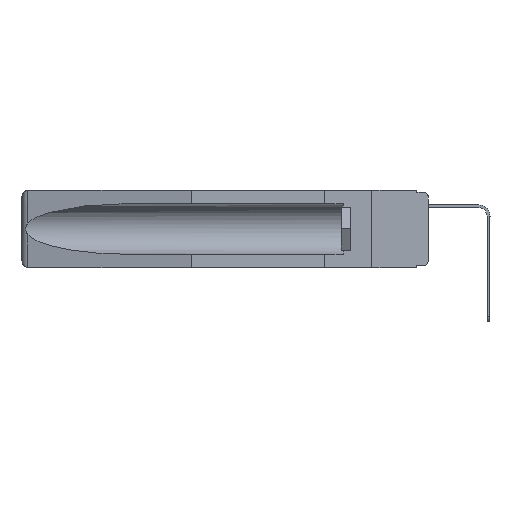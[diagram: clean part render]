
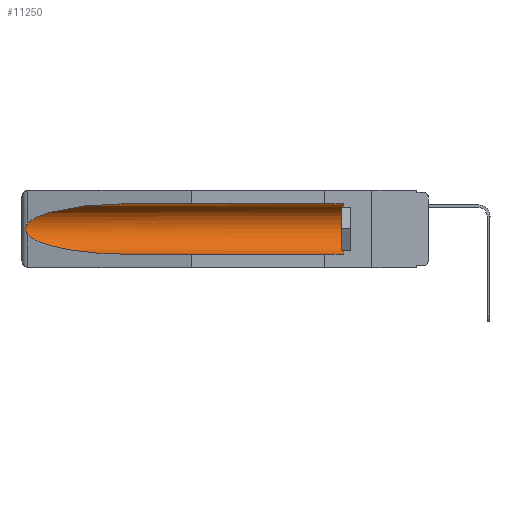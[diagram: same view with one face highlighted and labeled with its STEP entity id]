
A CAD part, left-side view. The second image highlights one B-rep face of the part: STEP entity #11250.
In plain terms, the highlighted cylindrical face has radius 2.857 mm (diameter 5.715 mm), a partial arc.
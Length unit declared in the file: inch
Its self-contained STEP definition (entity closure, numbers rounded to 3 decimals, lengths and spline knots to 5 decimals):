
#95 = EDGE_CURVE ( 'NONE', #7222, #11001, #99, .T. ) ;
#99 =( BOUNDED_CURVE ( )  B_SPLINE_CURVE ( 3, ( #16822, #16918, #8422, #4584 ),
 .UNSPECIFIED., .F., .F. ) 
 B_SPLINE_CURVE_WITH_KNOTS ( ( 4, 4 ),
 ( 4.71239, 6.08839 ),
 .UNSPECIFIED. ) 
 CURVE ( )  GEOMETRIC_REPRESENTATION_ITEM ( )  RATIONAL_B_SPLINE_CURVE ( ( 1., 0.848, 0.848, 1. ) ) 
 REPRESENTATION_ITEM ( '' )  );
#2267 = CARTESIAN_POINT ( 'NONE',  ( 0.155, 0.126, -0.1715 ) ) ;
#2500 = VECTOR ( 'NONE', #25527, 39.37008 ) ;
#2703 = DIRECTION ( 'NONE',  ( 0., 1., 0. ) ) ;
#2849 = CARTESIAN_POINT ( 'NONE',  ( 0.2673, 1.5327, -0.16383 ) ) ;
#3856 = ORIENTED_EDGE ( 'NONE', *, *, #95, .T. ) ;
#4128 = LINE ( 'NONE', #4716, #2500 ) ;
#4533 = EDGE_CURVE ( 'NONE', #25367, #26791, #5265, .T. ) ;
#4584 = CARTESIAN_POINT ( 'NONE',  ( 0.26537, 1.52718, -0.14972 ) ) ;
#4716 = CARTESIAN_POINT ( 'NONE',  ( 0.155, -0.30754, -0.059 ) ) ;
#4916 = CARTESIAN_POINT ( 'NONE',  ( 0.2675, 1.53308, -0.17534 ) ) ;
#5265 = LINE ( 'NONE', #25731, #25016 ) ;
#5566 = VERTEX_POINT ( 'NONE', #25139 ) ;
#6490 = EDGE_CURVE ( 'NONE', #25367, #23453, #13890, .T. ) ;
#7222 = VERTEX_POINT ( 'NONE', #23536 ) ;
#7542 = ORIENTED_EDGE ( 'NONE', *, *, #21500, .T. ) ;
#7669 = CARTESIAN_POINT ( 'NONE',  ( 0.25451, 1.48313, -0.24835 ) ) ;
#7683 = EDGE_CURVE ( 'NONE', #23453, #7222, #4128, .T. ) ;
#7862 = B_SPLINE_CURVE_WITH_KNOTS ( 'NONE', 3,
 ( #25556, #15195, #11122, #2849, #17074, #4916, #11203, #19445, #17253, #19168 ),
 .UNSPECIFIED., .F., .F.,
 ( 4, 2, 2, 2, 4 ),
 ( 0., 0.00029, 0.00058, 0.00087, 0.00117 ),
 .UNSPECIFIED. ) ;
#8422 = CARTESIAN_POINT ( 'NONE',  ( 0.25451, 1.48313, -0.09465 ) ) ;
#8702 = CARTESIAN_POINT ( 'NONE',  ( 0.155, 1.07973, -0.284 ) ) ;
#10171 = AXIS2_PLACEMENT_3D ( 'NONE', #21479, #2703, #23297 ) ;
#10248 = ORIENTED_EDGE ( 'NONE', *, *, #4533, .F. ) ;
#11001 = VERTEX_POINT ( 'NONE', #16662 ) ;
#11111 = CARTESIAN_POINT ( 'NONE',  ( 0.155, 0.126, -0.059 ) ) ;
#11122 = CARTESIAN_POINT ( 'NONE',  ( 0.26654, 1.53092, -0.15636 ) ) ;
#11203 = CARTESIAN_POINT ( 'NONE',  ( 0.2673, 1.53269, -0.17917 ) ) ;
#11208 = EDGE_LOOP ( 'NONE', ( #3856, #7542, #13948, #10248, #24063, #21487 ) ) ;
#11250 = ADVANCED_FACE ( 'NONE', ( #21364 ), #20712, .F. ) ;
#11547 = CARTESIAN_POINT ( 'NONE',  ( 0.26537, 1.52718, -0.19328 ) ) ;
#13382 = AXIS2_PLACEMENT_3D ( 'NONE', #2267, #24197, #25681 ) ;
#13890 = CIRCLE ( 'NONE', #13382, 0.1125 ) ;
#13948 = ORIENTED_EDGE ( 'NONE', *, *, #26395, .T. ) ;
#15195 = CARTESIAN_POINT ( 'NONE',  ( 0.26597, 1.52961, -0.15275 ) ) ;
#15942 = CARTESIAN_POINT ( 'NONE',  ( 0.155, 0.126, -0.284 ) ) ;
#16662 = CARTESIAN_POINT ( 'NONE',  ( 0.26537, 1.52718, -0.14972 ) ) ;
#16822 = CARTESIAN_POINT ( 'NONE',  ( 0.155, 1.07973, -0.059 ) ) ;
#16918 = CARTESIAN_POINT ( 'NONE',  ( 0.21114, 1.30732, -0.059 ) ) ;
#17074 = CARTESIAN_POINT ( 'NONE',  ( 0.2675, 1.53308, -0.16763 ) ) ;
#17253 = CARTESIAN_POINT ( 'NONE',  ( 0.26597, 1.5296, -0.19026 ) ) ;
#17874 = CARTESIAN_POINT ( 'NONE',  ( 0.21114, 1.30732, -0.284 ) ) ;
#19168 = CARTESIAN_POINT ( 'NONE',  ( 0.26537, 1.52718, -0.19328 ) ) ;
#19445 = CARTESIAN_POINT ( 'NONE',  ( 0.26655, 1.53094, -0.18657 ) ) ;
#20712 = CYLINDRICAL_SURFACE ( 'NONE', #10171, 0.1125 ) ;
#21364 = FACE_OUTER_BOUND ( 'NONE', #11208, .T. ) ;
#21479 = CARTESIAN_POINT ( 'NONE',  ( 0.155, -0.30754, -0.1715 ) ) ;
#21487 = ORIENTED_EDGE ( 'NONE', *, *, #7683, .T. ) ;
#21500 = EDGE_CURVE ( 'NONE', #11001, #5566, #7862, .T. ) ;
#21810 = DIRECTION ( 'NONE',  ( 0., 1., 0. ) ) ;
#23297 = DIRECTION ( 'NONE',  ( 0., 0., 1. ) ) ;
#23453 = VERTEX_POINT ( 'NONE', #11111 ) ;
#23536 = CARTESIAN_POINT ( 'NONE',  ( 0.155, 1.07973, -0.059 ) ) ;
#24063 = ORIENTED_EDGE ( 'NONE', *, *, #6490, .T. ) ;
#24197 = DIRECTION ( 'NONE',  ( 0., -1., 0. ) ) ;
#25016 = VECTOR ( 'NONE', #21810, 39.37008 ) ;
#25139 = CARTESIAN_POINT ( 'NONE',  ( 0.26537, 1.52718, -0.19328 ) ) ;
#25367 = VERTEX_POINT ( 'NONE', #15942 ) ;
#25527 = DIRECTION ( 'NONE',  ( 0., 1., 0. ) ) ;
#25556 = CARTESIAN_POINT ( 'NONE',  ( 0.26537, 1.52718, -0.14972 ) ) ;
#25681 = DIRECTION ( 'NONE',  ( 0., 0., 1. ) ) ;
#25731 = CARTESIAN_POINT ( 'NONE',  ( 0.155, -0.30754, -0.284 ) ) ;
#26072 = CARTESIAN_POINT ( 'NONE',  ( 0.155, 1.07973, -0.284 ) ) ;
#26342 =( BOUNDED_CURVE ( )  B_SPLINE_CURVE ( 3, ( #11547, #7669, #17874, #26072 ),
 .UNSPECIFIED., .F., .F. ) 
 B_SPLINE_CURVE_WITH_KNOTS ( ( 4, 4 ),
 ( 0.1948, 1.5708 ),
 .UNSPECIFIED. ) 
 CURVE ( )  GEOMETRIC_REPRESENTATION_ITEM ( )  RATIONAL_B_SPLINE_CURVE ( ( 1., 0.848, 0.848, 1. ) ) 
 REPRESENTATION_ITEM ( '' )  );
#26395 = EDGE_CURVE ( 'NONE', #5566, #26791, #26342, .T. ) ;
#26791 = VERTEX_POINT ( 'NONE', #8702 ) ;
